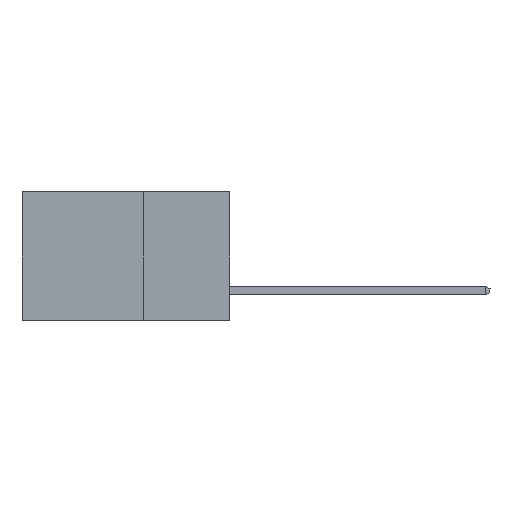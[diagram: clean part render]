
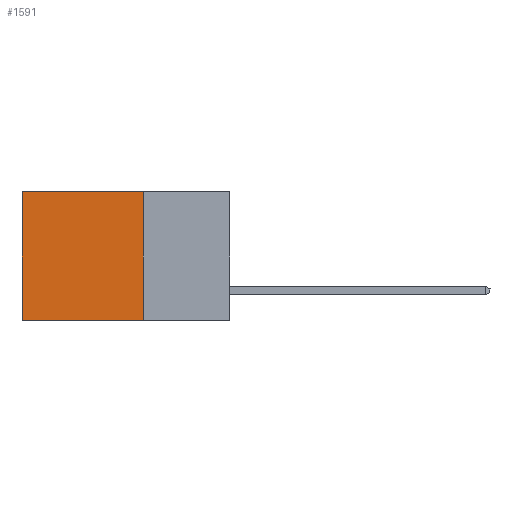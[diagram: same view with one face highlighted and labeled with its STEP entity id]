
A CAD part, left-side view. The second image highlights one B-rep face of the part: STEP entity #1591.
In plain terms, the highlighted planar face has unit normal (-1, 0, 0).
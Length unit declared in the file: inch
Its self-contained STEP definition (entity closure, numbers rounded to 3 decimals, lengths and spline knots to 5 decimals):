
#926 = VERTEX_POINT ( 'NONE', #18406 ) ;
#1591 = ADVANCED_FACE ( 'NONE', ( #13777 ), #10362, .F. ) ;
#1657 = ORIENTED_EDGE ( 'NONE', *, *, #2318, .T. ) ;
#2254 = DIRECTION ( 'NONE',  ( 0., 1., 0. ) ) ;
#2318 = EDGE_CURVE ( 'NONE', #18633, #16109, #4114, .T. ) ;
#2434 = ORIENTED_EDGE ( 'NONE', *, *, #11327, .F. ) ;
#2723 = CARTESIAN_POINT ( 'NONE',  ( 0.2615, 0.25, -0.37 ) ) ;
#4114 = LINE ( 'NONE', #7161, #14131 ) ;
#4597 = ORIENTED_EDGE ( 'NONE', *, *, #7610, .T. ) ;
#5477 = CARTESIAN_POINT ( 'NONE',  ( 0.2615, 0.25, -0.37 ) ) ;
#6760 = LINE ( 'NONE', #5477, #16129 ) ;
#7013 = LINE ( 'NONE', #17095, #7575 ) ;
#7161 = CARTESIAN_POINT ( 'NONE',  ( 0.2615, 0.25, 0. ) ) ;
#7575 = VECTOR ( 'NONE', #9416, 39.37008 ) ;
#7610 = EDGE_CURVE ( 'NONE', #16109, #926, #9503, .T. ) ;
#8511 = EDGE_LOOP ( 'NONE', ( #4597, #14397, #2434, #1657 ) ) ;
#9416 = DIRECTION ( 'NONE',  ( 0., 0., -1. ) ) ;
#9503 = LINE ( 'NONE', #12527, #11311 ) ;
#10362 = PLANE ( 'NONE',  #15391 ) ;
#10479 = CARTESIAN_POINT ( 'NONE',  ( 0.2615, 0.25, -0.37 ) ) ;
#10931 = CARTESIAN_POINT ( 'NONE',  ( 0.2615, 0.6, 0. ) ) ;
#11311 = VECTOR ( 'NONE', #16698, 39.37008 ) ;
#11327 = EDGE_CURVE ( 'NONE', #18633, #17489, #7013, .T. ) ;
#12527 = CARTESIAN_POINT ( 'NONE',  ( 0.2615, 0.6, -0.37 ) ) ;
#13313 = DIRECTION ( 'NONE',  ( 0., 0., -1. ) ) ;
#13738 = CARTESIAN_POINT ( 'NONE',  ( 0.2615, 0.25, 0. ) ) ;
#13777 = FACE_OUTER_BOUND ( 'NONE', #8511, .T. ) ;
#14131 = VECTOR ( 'NONE', #2254, 39.37008 ) ;
#14228 = EDGE_CURVE ( 'NONE', #17489, #926, #6760, .T. ) ;
#14397 = ORIENTED_EDGE ( 'NONE', *, *, #14228, .F. ) ;
#15391 = AXIS2_PLACEMENT_3D ( 'NONE', #2723, #17777, #13313 ) ;
#16100 = DIRECTION ( 'NONE',  ( 0., 1., 0. ) ) ;
#16109 = VERTEX_POINT ( 'NONE', #10931 ) ;
#16129 = VECTOR ( 'NONE', #16100, 39.37008 ) ;
#16698 = DIRECTION ( 'NONE',  ( 0., 0., -1. ) ) ;
#17095 = CARTESIAN_POINT ( 'NONE',  ( 0.2615, 0.25, -0.37 ) ) ;
#17489 = VERTEX_POINT ( 'NONE', #10479 ) ;
#17777 = DIRECTION ( 'NONE',  ( 1., 0., 0. ) ) ;
#18406 = CARTESIAN_POINT ( 'NONE',  ( 0.2615, 0.6, -0.37 ) ) ;
#18633 = VERTEX_POINT ( 'NONE', #13738 ) ;
